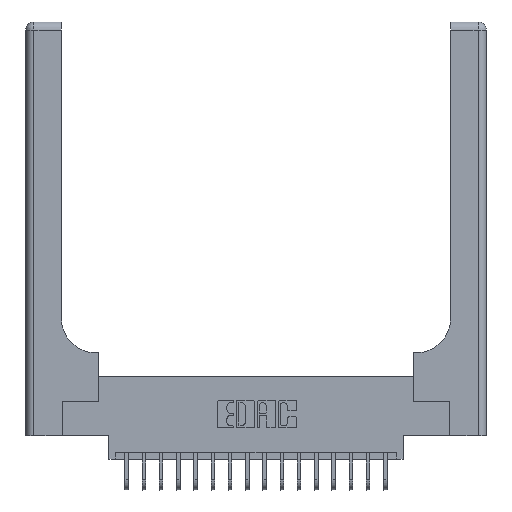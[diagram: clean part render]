
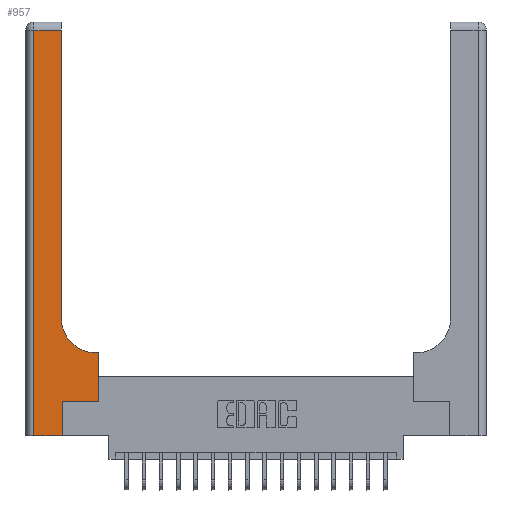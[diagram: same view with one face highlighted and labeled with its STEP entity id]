
A CAD part, top view. The second image highlights one B-rep face of the part: STEP entity #957.
In plain terms, the highlighted planar face has unit normal (0, 0, 1).
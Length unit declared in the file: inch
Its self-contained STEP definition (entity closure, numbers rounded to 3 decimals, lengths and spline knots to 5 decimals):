
#97 = CARTESIAN_POINT ( 'NONE',  ( 0.51, 0.6, 0.37 ) ) ;
#253 = VERTEX_POINT ( 'NONE', #10266 ) ;
#298 = VECTOR ( 'NONE', #15097, 39.37008 ) ;
#889 = VECTOR ( 'NONE', #8477, 39.37008 ) ;
#950 = CARTESIAN_POINT ( 'NONE',  ( 0.528, 0.25, 0.37 ) ) ;
#957 = ADVANCED_FACE ( 'NONE', ( #6618 ), #19488, .F. ) ;
#1400 = DIRECTION ( 'NONE',  ( -1., 0., 0. ) ) ;
#1477 = VERTEX_POINT ( 'NONE', #97 ) ;
#1818 = DIRECTION ( 'NONE',  ( -1., 0., 0. ) ) ;
#2198 = LINE ( 'NONE', #2313, #5417 ) ;
#2299 = EDGE_CURVE ( 'NONE', #12839, #14795, #18391, .T. ) ;
#2313 = CARTESIAN_POINT ( 'NONE',  ( 0.265, 0., 0.37 ) ) ;
#2368 = CARTESIAN_POINT ( 'NONE',  ( 0.06, 2.94, 0.37 ) ) ;
#2426 = LINE ( 'NONE', #17443, #4911 ) ;
#3253 = CARTESIAN_POINT ( 'NONE',  ( 0.265, 0.25, 0.37 ) ) ;
#3513 = ORIENTED_EDGE ( 'NONE', *, *, #13876, .T. ) ;
#3611 = EDGE_CURVE ( 'NONE', #14795, #20633, #2198, .T. ) ;
#3652 = CARTESIAN_POINT ( 'NONE',  ( 0.26, 0.6, 0.37 ) ) ;
#3829 = VERTEX_POINT ( 'NONE', #16293 ) ;
#3932 = EDGE_CURVE ( 'NONE', #20467, #253, #17156, .T. ) ;
#4145 = ORIENTED_EDGE ( 'NONE', *, *, #3611, .T. ) ;
#4224 = AXIS2_PLACEMENT_3D ( 'NONE', #19708, #4569, #16427 ) ;
#4569 = DIRECTION ( 'NONE',  ( 0., 0., -1. ) ) ;
#4681 = VECTOR ( 'NONE', #20155, 39.37008 ) ;
#4743 = EDGE_LOOP ( 'NONE', ( #19457, #19231, #15919, #12078, #4145, #3513, #21354, #8924, #8263 ) ) ;
#4911 = VECTOR ( 'NONE', #15705, 39.37008 ) ;
#5283 = EDGE_CURVE ( 'NONE', #253, #14495, #16295, .T. ) ;
#5417 = VECTOR ( 'NONE', #8933, 39.37008 ) ;
#6356 = DIRECTION ( 'NONE',  ( 0., 0., -1. ) ) ;
#6618 = FACE_OUTER_BOUND ( 'NONE', #4743, .T. ) ;
#7136 = LINE ( 'NONE', #3652, #14836 ) ;
#7370 = CARTESIAN_POINT ( 'NONE',  ( 0.528, 0.6, 0.37 ) ) ;
#7784 = VERTEX_POINT ( 'NONE', #7370 ) ;
#8095 = DIRECTION ( 'NONE',  ( 1., 0., 0. ) ) ;
#8263 = ORIENTED_EDGE ( 'NONE', *, *, #9667, .T. ) ;
#8477 = DIRECTION ( 'NONE',  ( 1., 0., 0. ) ) ;
#8557 = CARTESIAN_POINT ( 'NONE',  ( 0.26, 3., 0.37 ) ) ;
#8924 = ORIENTED_EDGE ( 'NONE', *, *, #16076, .T. ) ;
#8933 = DIRECTION ( 'NONE',  ( 0., 1., 0. ) ) ;
#9003 = CARTESIAN_POINT ( 'NONE',  ( 0.26, 0.85, 0.37 ) ) ;
#9667 = EDGE_CURVE ( 'NONE', #1477, #20467, #18865, .T. ) ;
#10266 = CARTESIAN_POINT ( 'NONE',  ( 0.26, 2.94, 0.37 ) ) ;
#10542 = LINE ( 'NONE', #17190, #4681 ) ;
#10571 = CARTESIAN_POINT ( 'NONE',  ( 0.265, 0., 0.37 ) ) ;
#11516 = CARTESIAN_POINT ( 'NONE',  ( 0., 2.94, 0.37 ) ) ;
#11741 = VECTOR ( 'NONE', #20960, 39.37008 ) ;
#12078 = ORIENTED_EDGE ( 'NONE', *, *, #2299, .T. ) ;
#12839 = VERTEX_POINT ( 'NONE', #19234 ) ;
#13314 = AXIS2_PLACEMENT_3D ( 'NONE', #21278, #6356, #8095 ) ;
#13876 = EDGE_CURVE ( 'NONE', #20633, #3829, #10542, .T. ) ;
#14495 = VERTEX_POINT ( 'NONE', #2368 ) ;
#14629 = LINE ( 'NONE', #950, #11741 ) ;
#14795 = VERTEX_POINT ( 'NONE', #10571 ) ;
#14836 = VECTOR ( 'NONE', #1818, 39.37008 ) ;
#15097 = DIRECTION ( 'NONE',  ( 0., 1., 0. ) ) ;
#15296 = VECTOR ( 'NONE', #1400, 39.37008 ) ;
#15705 = DIRECTION ( 'NONE',  ( 0., -1., 0. ) ) ;
#15919 = ORIENTED_EDGE ( 'NONE', *, *, #21184, .T. ) ;
#16076 = EDGE_CURVE ( 'NONE', #7784, #1477, #7136, .T. ) ;
#16293 = CARTESIAN_POINT ( 'NONE',  ( 0.528, 0.25, 0.37 ) ) ;
#16295 = LINE ( 'NONE', #11516, #15296 ) ;
#16427 = DIRECTION ( 'NONE',  ( -1., 0., 0. ) ) ;
#17156 = LINE ( 'NONE', #8557, #298 ) ;
#17190 = CARTESIAN_POINT ( 'NONE',  ( 0.265, 0.25, 0.37 ) ) ;
#17443 = CARTESIAN_POINT ( 'NONE',  ( 0.06, 3., 0.37 ) ) ;
#17947 = EDGE_CURVE ( 'NONE', #3829, #7784, #14629, .T. ) ;
#18391 = LINE ( 'NONE', #20253, #889 ) ;
#18865 = CIRCLE ( 'NONE', #13314, 0.25 ) ;
#19231 = ORIENTED_EDGE ( 'NONE', *, *, #5283, .T. ) ;
#19234 = CARTESIAN_POINT ( 'NONE',  ( 0.06, 0., 0.37 ) ) ;
#19457 = ORIENTED_EDGE ( 'NONE', *, *, #3932, .T. ) ;
#19488 = PLANE ( 'NONE',  #4224 ) ;
#19708 = CARTESIAN_POINT ( 'NONE',  ( 0., 3., 0.37 ) ) ;
#20155 = DIRECTION ( 'NONE',  ( 1., 0., 0. ) ) ;
#20253 = CARTESIAN_POINT ( 'NONE',  ( 0., 0., 0.37 ) ) ;
#20467 = VERTEX_POINT ( 'NONE', #9003 ) ;
#20633 = VERTEX_POINT ( 'NONE', #3253 ) ;
#20960 = DIRECTION ( 'NONE',  ( 0., 1., 0. ) ) ;
#21184 = EDGE_CURVE ( 'NONE', #14495, #12839, #2426, .T. ) ;
#21278 = CARTESIAN_POINT ( 'NONE',  ( 0.51, 0.85, 0.37 ) ) ;
#21354 = ORIENTED_EDGE ( 'NONE', *, *, #17947, .T. ) ;
